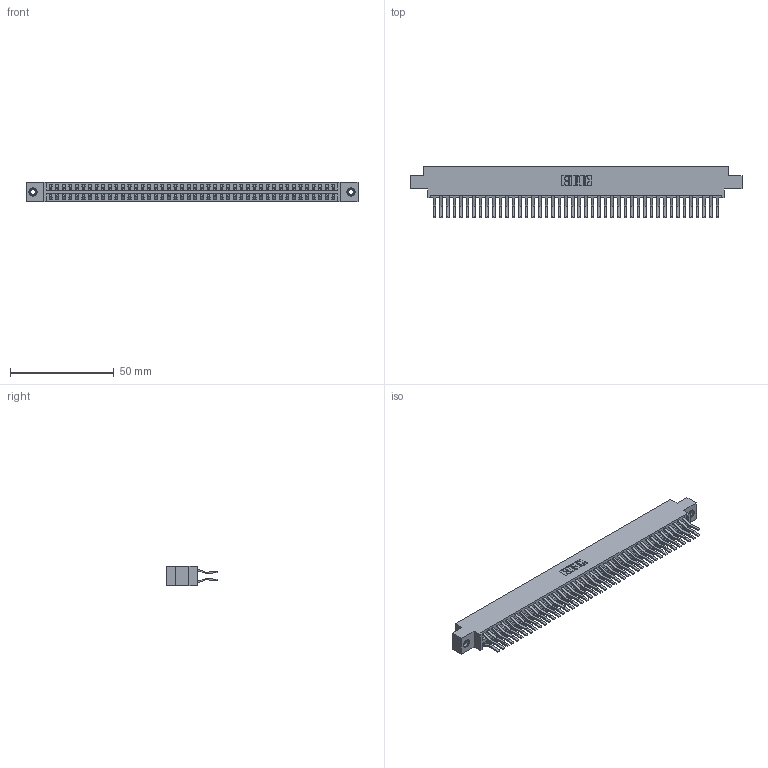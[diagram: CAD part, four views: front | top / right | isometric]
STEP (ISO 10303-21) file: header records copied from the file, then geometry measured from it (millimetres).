
FILE_DESCRIPTION (( 'STEP AP203' ), '1' );
FILE_NAME ('396-088-560-807.STEP', '2019-11-02T15:19:35', ( '' ), ( '' ), 'SwSTEP 2.0', 'SolidWorks 2016', '' );
FILE_SCHEMA (( 'CONFIG_CONTROL_DESIGN' ));
Length unit declared in the file: inch
Products named in the file (4): 345-292-001_560 Tail; 345-250-001_345-250-005-103; 396-088-560-807; 346 Part_0.170 Offset - 0.156 Dia-TI
Assembly tree (91 placements, depth 2):
  396-088-560-807
    346 Part_0.170 Offset - 0.156 Dia-TI
    345-292-001_560 Tail  x88
    345-250-001_345-250-005-103  x2
Bounding box: 160.27 x 24.78 x 9.4 mm (x, y, z)
Volume: 16052.9 mm3; surface area: 23849.5 mm2
Topology: 91 solids, 91 shells, 4938 faces, 14645 edges, 9638 vertices
Faces by surface type: plane 3192, cylinder 1730, cone 12, torus 4
Entity records: 29852 total; most frequent: CARTESIAN_POINT 4903, ORIENTED_EDGE 4830, DIRECTION 4401, EDGE_CURVE 2415, VECTOR 2083, LINE 2083, VERTEX_POINT 1604, AXIS2_PLACEMENT_3D 1159
